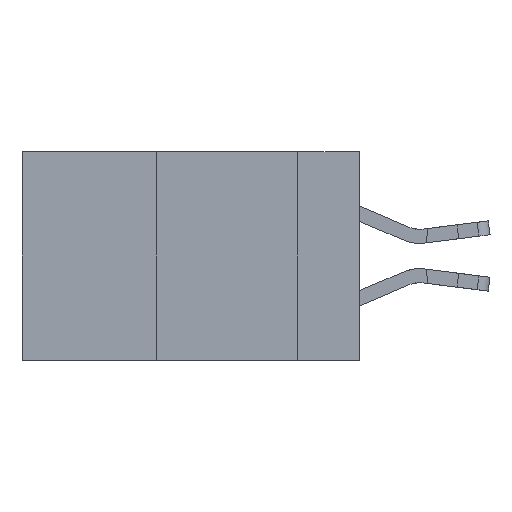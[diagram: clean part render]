
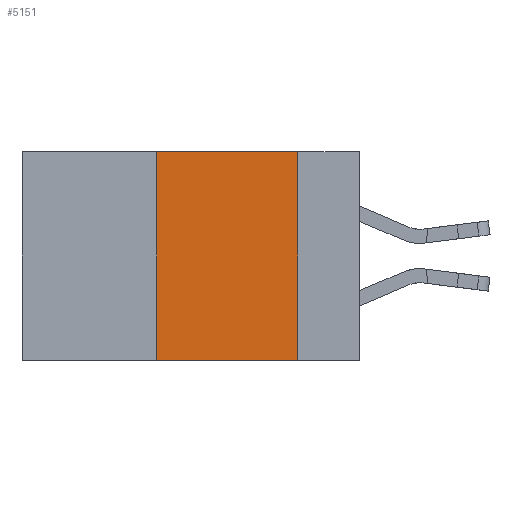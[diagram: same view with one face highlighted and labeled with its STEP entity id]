
A CAD part, left-side view. The second image highlights one B-rep face of the part: STEP entity #5151.
In plain terms, the highlighted planar face has unit normal (-1, 0, 0).
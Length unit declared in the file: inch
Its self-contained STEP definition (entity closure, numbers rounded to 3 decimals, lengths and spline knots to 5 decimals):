
#217 = CARTESIAN_POINT ( 'NONE',  ( 0., 0.36, 0. ) ) ;
#538 = ORIENTED_EDGE ( 'NONE', *, *, #15809, .F. ) ;
#551 = LINE ( 'NONE', #2184, #15796 ) ;
#676 = DIRECTION ( 'NONE',  ( 0., -1., 0. ) ) ;
#749 = CARTESIAN_POINT ( 'NONE',  ( 0., 0.6, 0. ) ) ;
#1933 = LINE ( 'NONE', #16569, #14074 ) ;
#2184 = CARTESIAN_POINT ( 'NONE',  ( 0., 0.11, 0. ) ) ;
#2237 = DIRECTION ( 'NONE',  ( 0., -1., 0. ) ) ;
#3573 = LINE ( 'NONE', #15254, #11885 ) ;
#3809 = FACE_OUTER_BOUND ( 'NONE', #13469, .T. ) ;
#4613 = EDGE_CURVE ( 'NONE', #18361, #6038, #1933, .T. ) ;
#4894 = EDGE_CURVE ( 'NONE', #6950, #18361, #11769, .T. ) ;
#5151 = ADVANCED_FACE ( 'NONE', ( #3809 ), #6866, .F. ) ;
#5526 = DIRECTION ( 'NONE',  ( 0., 0., -1. ) ) ;
#6017 = DIRECTION ( 'NONE',  ( 0., 0., 1. ) ) ;
#6038 = VERTEX_POINT ( 'NONE', #14652 ) ;
#6866 = PLANE ( 'NONE',  #8886 ) ;
#6909 = VERTEX_POINT ( 'NONE', #12207 ) ;
#6950 = VERTEX_POINT ( 'NONE', #10854 ) ;
#7336 = VECTOR ( 'NONE', #6017, 39.37008 ) ;
#7454 = CARTESIAN_POINT ( 'NONE',  ( 0., 0.36, 0. ) ) ;
#8886 = AXIS2_PLACEMENT_3D ( 'NONE', #749, #12814, #5526 ) ;
#10854 = CARTESIAN_POINT ( 'NONE',  ( 0., 0.36, -0.37 ) ) ;
#11769 = LINE ( 'NONE', #7454, #7336 ) ;
#11885 = VECTOR ( 'NONE', #2237, 39.37008 ) ;
#12207 = CARTESIAN_POINT ( 'NONE',  ( 0., 0.11, -0.37 ) ) ;
#12814 = DIRECTION ( 'NONE',  ( 1., 0., 0. ) ) ;
#13469 = EDGE_LOOP ( 'NONE', ( #538, #15630, #18561, #15471 ) ) ;
#14074 = VECTOR ( 'NONE', #676, 39.37008 ) ;
#14652 = CARTESIAN_POINT ( 'NONE',  ( 0., 0.11, 0. ) ) ;
#15254 = CARTESIAN_POINT ( 'NONE',  ( 0., 0.6, -0.37 ) ) ;
#15471 = ORIENTED_EDGE ( 'NONE', *, *, #17921, .T. ) ;
#15630 = ORIENTED_EDGE ( 'NONE', *, *, #4613, .F. ) ;
#15796 = VECTOR ( 'NONE', #18169, 39.37008 ) ;
#15809 = EDGE_CURVE ( 'NONE', #6038, #6909, #551, .T. ) ;
#16569 = CARTESIAN_POINT ( 'NONE',  ( 0., 0.6, 0. ) ) ;
#17921 = EDGE_CURVE ( 'NONE', #6950, #6909, #3573, .T. ) ;
#18169 = DIRECTION ( 'NONE',  ( 0., 0., -1. ) ) ;
#18361 = VERTEX_POINT ( 'NONE', #217 ) ;
#18561 = ORIENTED_EDGE ( 'NONE', *, *, #4894, .F. ) ;
